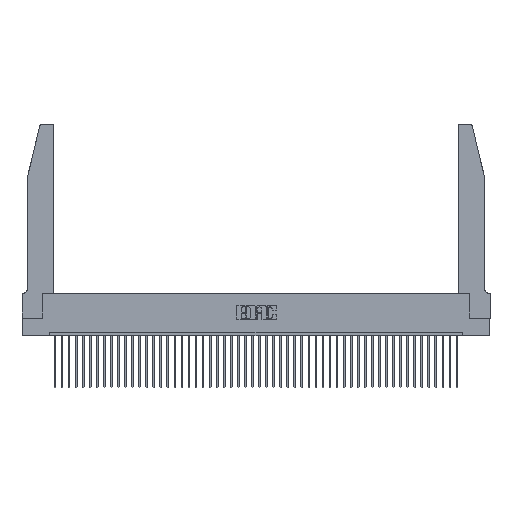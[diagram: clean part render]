
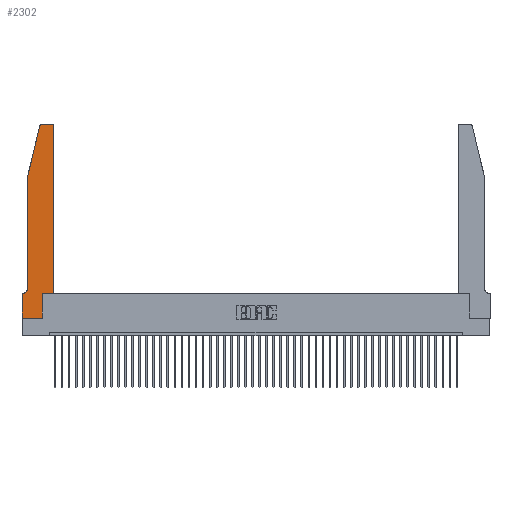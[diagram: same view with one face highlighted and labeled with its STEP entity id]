
A CAD part, top view. The second image highlights one B-rep face of the part: STEP entity #2302.
In plain terms, the highlighted planar face has unit normal (0, 0, 1).
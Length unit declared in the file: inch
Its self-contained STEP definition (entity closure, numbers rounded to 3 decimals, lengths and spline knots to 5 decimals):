
#1028 = ORIENTED_EDGE ( 'NONE', *, *, #42332, .T. ) ;
#1312 = VERTEX_POINT ( 'NONE', #16190 ) ;
#1442 = CARTESIAN_POINT ( 'NONE',  ( 0.0755, 2., 0.37 ) ) ;
#2280 = FACE_OUTER_BOUND ( 'NONE', #33657, .T. ) ;
#2302 = ADVANCED_FACE ( 'NONE', ( #2280 ), #39720, .T. ) ;
#2405 = DIRECTION ( 'NONE',  ( -1., 0., 0. ) ) ;
#2611 = AXIS2_PLACEMENT_3D ( 'NONE', #40489, #8535, #44087 ) ;
#2806 = CARTESIAN_POINT ( 'NONE',  ( 0.0755, 2., 0.37 ) ) ;
#3002 = ORIENTED_EDGE ( 'NONE', *, *, #10880, .T. ) ;
#3008 = VERTEX_POINT ( 'NONE', #40404 ) ;
#3720 = CARTESIAN_POINT ( 'NONE',  ( 0.2865, 0.35, 0.37 ) ) ;
#3832 = CARTESIAN_POINT ( 'NONE',  ( 0., 0.35, 0.37 ) ) ;
#4068 = ORIENTED_EDGE ( 'NONE', *, *, #31789, .T. ) ;
#4115 = VECTOR ( 'NONE', #45867, 39.37008 ) ;
#4478 = CARTESIAN_POINT ( 'NONE',  ( 0.4505, 2.72, 0.37 ) ) ;
#5350 = CIRCLE ( 'NONE', #2611, 0.07 ) ;
#5369 = CARTESIAN_POINT ( 'NONE',  ( 0.2865, 0., 0.37 ) ) ;
#5697 = VECTOR ( 'NONE', #22582, 39.37008 ) ;
#8254 = CARTESIAN_POINT ( 'NONE',  ( 0.4205, 2.75, 0.37 ) ) ;
#8257 = VERTEX_POINT ( 'NONE', #29163 ) ;
#8290 = ORIENTED_EDGE ( 'NONE', *, *, #34788, .T. ) ;
#8372 = CARTESIAN_POINT ( 'NONE',  ( 0.0755, 2., 0.37 ) ) ;
#8535 = DIRECTION ( 'NONE',  ( 0., 0., -1. ) ) ;
#8839 = AXIS2_PLACEMENT_3D ( 'NONE', #45119, #39010, #33317 ) ;
#9552 = VECTOR ( 'NONE', #29483, 39.37008 ) ;
#10495 = CARTESIAN_POINT ( 'NONE',  ( 0.284, 2.72, 0.37 ) ) ;
#10533 = DIRECTION ( 'NONE',  ( -1., 0., 0. ) ) ;
#10638 = EDGE_CURVE ( 'NONE', #38354, #22735, #33481, .T. ) ;
#10668 = EDGE_CURVE ( 'NONE', #14862, #14466, #22885, .T. ) ;
#10880 = EDGE_CURVE ( 'NONE', #26116, #28081, #28512, .T. ) ;
#11809 = EDGE_CURVE ( 'NONE', #22735, #33426, #30088, .T. ) ;
#12769 = CARTESIAN_POINT ( 'NONE',  ( 0.4505, 0.35, 0.37 ) ) ;
#12777 = VECTOR ( 'NONE', #40823, 39.37008 ) ;
#13044 = ORIENTED_EDGE ( 'NONE', *, *, #41239, .T. ) ;
#13738 = LINE ( 'NONE', #27943, #4115 ) ;
#14236 = CARTESIAN_POINT ( 'NONE',  ( 0.4505, 0.35, 0.37 ) ) ;
#14466 = VERTEX_POINT ( 'NONE', #35207 ) ;
#14862 = VERTEX_POINT ( 'NONE', #38799 ) ;
#15646 = VECTOR ( 'NONE', #31872, 39.37008 ) ;
#16190 = CARTESIAN_POINT ( 'NONE',  ( 0.25487, 2.72718, 0.37 ) ) ;
#16438 = EDGE_CURVE ( 'NONE', #33426, #3008, #46282, .T. ) ;
#16689 = EDGE_CURVE ( 'NONE', #14466, #29133, #22790, .T. ) ;
#17692 = ORIENTED_EDGE ( 'NONE', *, *, #10668, .T. ) ;
#17847 = CARTESIAN_POINT ( 'NONE',  ( 0.0755, 0.35, 0.37 ) ) ;
#19686 = CIRCLE ( 'NONE', #27771, 0.03 ) ;
#20629 = DIRECTION ( 'NONE',  ( 0., 0., 1. ) ) ;
#20651 = DIRECTION ( 'NONE',  ( 0., -1., 0. ) ) ;
#21134 = VECTOR ( 'NONE', #20651, 39.37008 ) ;
#21963 = DIRECTION ( 'NONE',  ( 1., 0., 0. ) ) ;
#22479 = VERTEX_POINT ( 'NONE', #2806 ) ;
#22582 = DIRECTION ( 'NONE',  ( 0., -1., 0. ) ) ;
#22735 = VERTEX_POINT ( 'NONE', #4478 ) ;
#22790 = LINE ( 'NONE', #27674, #21134 ) ;
#22885 = LINE ( 'NONE', #17847, #45255 ) ;
#23839 = CARTESIAN_POINT ( 'NONE',  ( 0.2605, 2.75, 0.37 ) ) ;
#24483 = LINE ( 'NONE', #8372, #12777 ) ;
#25144 = ORIENTED_EDGE ( 'NONE', *, *, #11809, .T. ) ;
#25588 = ORIENTED_EDGE ( 'NONE', *, *, #10638, .T. ) ;
#25662 = VECTOR ( 'NONE', #33764, 39.37008 ) ;
#26116 = VERTEX_POINT ( 'NONE', #5369 ) ;
#26121 = CARTESIAN_POINT ( 'NONE',  ( 0., 0., 0.37 ) ) ;
#27674 = CARTESIAN_POINT ( 'NONE',  ( 0., 0., 0.37 ) ) ;
#27771 = AXIS2_PLACEMENT_3D ( 'NONE', #10495, #20629, #34958 ) ;
#27943 = CARTESIAN_POINT ( 'NONE',  ( 0., 0., 0.37 ) ) ;
#28081 = VERTEX_POINT ( 'NONE', #3720 ) ;
#28268 = CARTESIAN_POINT ( 'NONE',  ( 0.4505, 0.35, 0.37 ) ) ;
#28512 = LINE ( 'NONE', #32430, #9552 ) ;
#28778 = ORIENTED_EDGE ( 'NONE', *, *, #16438, .T. ) ;
#29018 = DIRECTION ( 'NONE',  ( 0., 0., 1. ) ) ;
#29133 = VERTEX_POINT ( 'NONE', #26121 ) ;
#29163 = CARTESIAN_POINT ( 'NONE',  ( 0.0755, 0.42, 0.37 ) ) ;
#29483 = DIRECTION ( 'NONE',  ( 0., 1., 0. ) ) ;
#30088 = CIRCLE ( 'NONE', #8839, 0.03 ) ;
#31789 = EDGE_CURVE ( 'NONE', #8257, #14862, #5350, .T. ) ;
#31841 = ORIENTED_EDGE ( 'NONE', *, *, #36805, .T. ) ;
#31872 = DIRECTION ( 'NONE',  ( 0., 1., 0. ) ) ;
#32430 = CARTESIAN_POINT ( 'NONE',  ( 0.2865, 0.35, 0.37 ) ) ;
#33317 = DIRECTION ( 'NONE',  ( 1., 0., 0. ) ) ;
#33426 = VERTEX_POINT ( 'NONE', #8254 ) ;
#33481 = LINE ( 'NONE', #14236, #15646 ) ;
#33657 = EDGE_LOOP ( 'NONE', ( #28778, #13044, #36306, #31841, #4068, #17692, #42636, #8290, #3002, #1028, #25588, #25144 ) ) ;
#33764 = DIRECTION ( 'NONE',  ( 1., 0., 0. ) ) ;
#34788 = EDGE_CURVE ( 'NONE', #29133, #26116, #13738, .T. ) ;
#34958 = DIRECTION ( 'NONE',  ( 1., 0., 0. ) ) ;
#35207 = CARTESIAN_POINT ( 'NONE',  ( 0., 0.35, 0.37 ) ) ;
#35345 = AXIS2_PLACEMENT_3D ( 'NONE', #3832, #29018, #21963 ) ;
#36306 = ORIENTED_EDGE ( 'NONE', *, *, #43375, .T. ) ;
#36805 = EDGE_CURVE ( 'NONE', #22479, #8257, #40842, .T. ) ;
#38354 = VERTEX_POINT ( 'NONE', #28268 ) ;
#38799 = CARTESIAN_POINT ( 'NONE',  ( 0.0055, 0.35, 0.37 ) ) ;
#39010 = DIRECTION ( 'NONE',  ( 0., 0., 1. ) ) ;
#39720 = PLANE ( 'NONE',  #35345 ) ;
#40404 = CARTESIAN_POINT ( 'NONE',  ( 0.284, 2.75, 0.37 ) ) ;
#40489 = CARTESIAN_POINT ( 'NONE',  ( 0.0055, 0.42, 0.37 ) ) ;
#40823 = DIRECTION ( 'NONE',  ( -0.239, -0.971, 0. ) ) ;
#40842 = LINE ( 'NONE', #1442, #5697 ) ;
#41239 = EDGE_CURVE ( 'NONE', #3008, #1312, #19686, .T. ) ;
#41258 = VECTOR ( 'NONE', #2405, 39.37008 ) ;
#42332 = EDGE_CURVE ( 'NONE', #28081, #38354, #44690, .T. ) ;
#42636 = ORIENTED_EDGE ( 'NONE', *, *, #16689, .T. ) ;
#43375 = EDGE_CURVE ( 'NONE', #1312, #22479, #24483, .T. ) ;
#44087 = DIRECTION ( 'NONE',  ( -1., 0., 0. ) ) ;
#44690 = LINE ( 'NONE', #12769, #25662 ) ;
#45119 = CARTESIAN_POINT ( 'NONE',  ( 0.4205, 2.72, 0.37 ) ) ;
#45255 = VECTOR ( 'NONE', #10533, 39.37008 ) ;
#45867 = DIRECTION ( 'NONE',  ( 1., 0., 0. ) ) ;
#46282 = LINE ( 'NONE', #23839, #41258 ) ;
